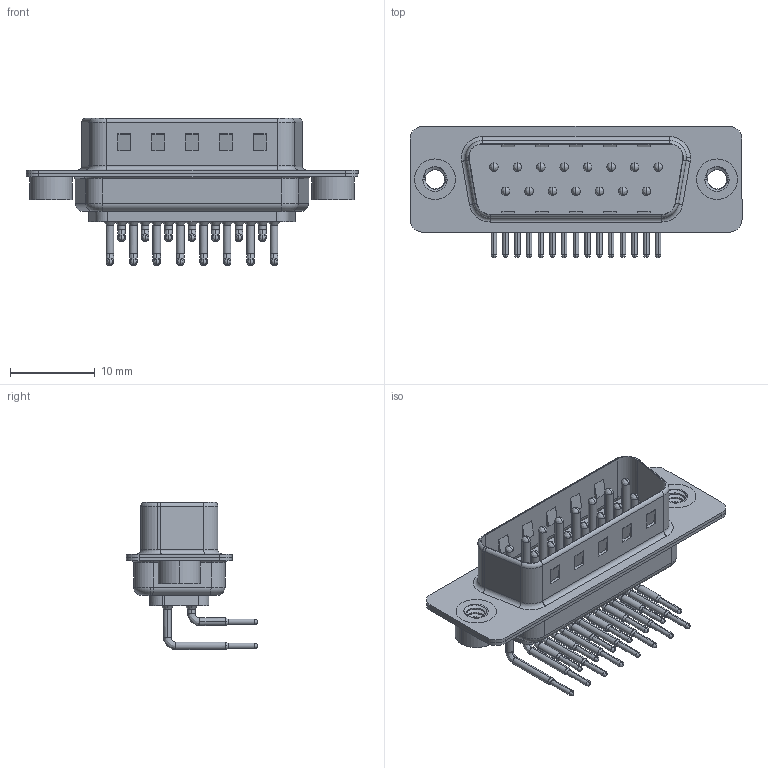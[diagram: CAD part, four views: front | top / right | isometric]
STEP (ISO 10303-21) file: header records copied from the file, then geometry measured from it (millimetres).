
FILE_DESCRIPTION (( 'STEP AP203' ), '1' );
FILE_NAME ('621-M15-660-LN2.STEP', '2018-09-25T00:58:00', ( '' ), ( '' ), 'SwSTEP 2.0', 'SolidWorks 2016', '' );
FILE_SCHEMA (( 'CONFIG_CONTROL_DESIGN' ));
Length unit declared in the file: millimetre
Products named in the file (7): 621M 4-40 Threaded Rivet; 621-M15-660-LN2; 621M Housing_15 Contacts; 621M Shell Front_15 Contacts; 621M Shell Rear_15 Contacts; 621M Contact Row 1; 621M Contact Row 2
Assembly tree (20 placements, depth 2):
  621-M15-660-LN2
    621M Housing_15 Contacts
    621M Shell Front_15 Contacts
    621M Shell Rear_15 Contacts
    621M Contact Row 1  x8
    621M Contact Row 2  x7
    621M 4-40 Threaded Rivet  x2
Bounding box: 39.2 x 15.49 x 17.39 mm (x, y, z)
Volume: 1937.9 mm3; surface area: 5261.6 mm2
Topology: 20 solids, 20 shells, 1990 faces, 5525 edges, 3586 vertices
Faces by surface type: plane 1099, cylinder 673, bspline 96, cone 66, torus 56
Entity records: 22132 total; most frequent: CARTESIAN_POINT 5074, DIRECTION 3467, ORIENTED_EDGE 3250, EDGE_CURVE 1625, AXIS2_PLACEMENT_3D 1252, VERTEX_POINT 1049, VECTOR 963, LINE 963
